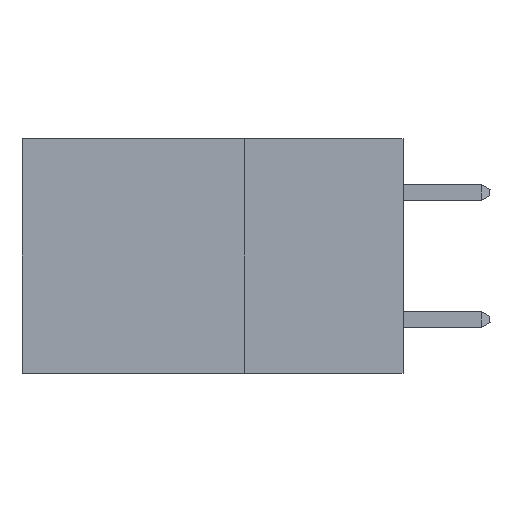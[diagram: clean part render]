
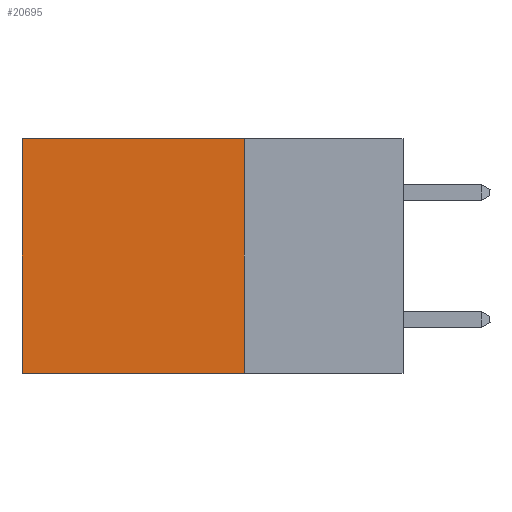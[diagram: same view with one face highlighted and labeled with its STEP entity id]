
A CAD part, left-side view. The second image highlights one B-rep face of the part: STEP entity #20695.
In plain terms, the highlighted planar face has unit normal (-1, 0, 0).
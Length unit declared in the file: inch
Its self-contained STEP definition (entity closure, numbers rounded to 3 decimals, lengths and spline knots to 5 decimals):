
#320 = VERTEX_POINT ( 'NONE', #26392 ) ;
#1510 = EDGE_CURVE ( 'NONE', #15818, #11219, #5323, .T. ) ;
#3877 = CARTESIAN_POINT ( 'NONE',  ( 0.2875, 0.25, 0. ) ) ;
#4852 = EDGE_CURVE ( 'NONE', #11219, #320, #15666, .T. ) ;
#5323 = LINE ( 'NONE', #33232, #34365 ) ;
#5360 = DIRECTION ( 'NONE',  ( 0., 1., 0. ) ) ;
#7472 = VECTOR ( 'NONE', #31917, 39.37008 ) ;
#8300 = FACE_OUTER_BOUND ( 'NONE', #19254, .T. ) ;
#11219 = VERTEX_POINT ( 'NONE', #36952 ) ;
#15217 = CARTESIAN_POINT ( 'NONE',  ( 0.2875, 0.25, -0.37 ) ) ;
#15510 = DIRECTION ( 'NONE',  ( 0., 0., -1. ) ) ;
#15666 = LINE ( 'NONE', #34894, #7472 ) ;
#15818 = VERTEX_POINT ( 'NONE', #28057 ) ;
#18267 = LINE ( 'NONE', #15217, #32355 ) ;
#18350 = DIRECTION ( 'NONE',  ( 0., 1., 0. ) ) ;
#19254 = EDGE_LOOP ( 'NONE', ( #28194, #28837, #22460, #24919 ) ) ;
#20669 = VERTEX_POINT ( 'NONE', #25142 ) ;
#20695 = ADVANCED_FACE ( 'NONE', ( #8300 ), #28387, .F. ) ;
#21919 = EDGE_CURVE ( 'NONE', #15818, #20669, #29584, .T. ) ;
#22460 = ORIENTED_EDGE ( 'NONE', *, *, #21919, .F. ) ;
#24919 = ORIENTED_EDGE ( 'NONE', *, *, #1510, .T. ) ;
#25008 = DIRECTION ( 'NONE',  ( 0., 0., -1. ) ) ;
#25138 = AXIS2_PLACEMENT_3D ( 'NONE', #3877, #37980, #25008 ) ;
#25142 = CARTESIAN_POINT ( 'NONE',  ( 0.2875, 0.25, -0.37 ) ) ;
#26392 = CARTESIAN_POINT ( 'NONE',  ( 0.2875, 0.6, -0.37 ) ) ;
#27632 = VECTOR ( 'NONE', #15510, 39.37008 ) ;
#28057 = CARTESIAN_POINT ( 'NONE',  ( 0.2875, 0.25, 0. ) ) ;
#28194 = ORIENTED_EDGE ( 'NONE', *, *, #4852, .T. ) ;
#28387 = PLANE ( 'NONE',  #25138 ) ;
#28837 = ORIENTED_EDGE ( 'NONE', *, *, #31780, .F. ) ;
#29584 = LINE ( 'NONE', #37611, #27632 ) ;
#31780 = EDGE_CURVE ( 'NONE', #20669, #320, #18267, .T. ) ;
#31917 = DIRECTION ( 'NONE',  ( 0., 0., -1. ) ) ;
#32355 = VECTOR ( 'NONE', #18350, 39.37008 ) ;
#33232 = CARTESIAN_POINT ( 'NONE',  ( 0.2875, 0.25, 0. ) ) ;
#34365 = VECTOR ( 'NONE', #5360, 39.37008 ) ;
#34894 = CARTESIAN_POINT ( 'NONE',  ( 0.2875, 0.6, 0. ) ) ;
#36952 = CARTESIAN_POINT ( 'NONE',  ( 0.2875, 0.6, 0. ) ) ;
#37611 = CARTESIAN_POINT ( 'NONE',  ( 0.2875, 0.25, 0. ) ) ;
#37980 = DIRECTION ( 'NONE',  ( 1., 0., 0. ) ) ;
